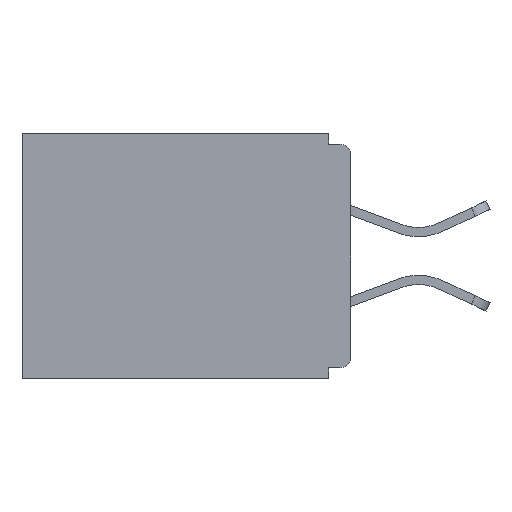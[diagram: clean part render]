
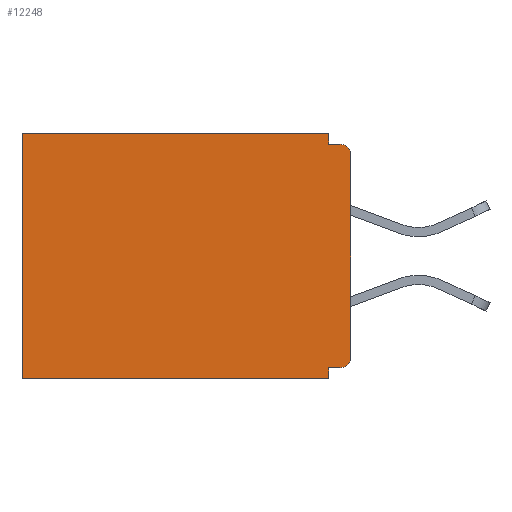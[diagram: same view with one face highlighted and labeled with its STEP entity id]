
A CAD part, left-side view. The second image highlights one B-rep face of the part: STEP entity #12248.
In plain terms, the highlighted planar face has unit normal (-1, 0, 0).
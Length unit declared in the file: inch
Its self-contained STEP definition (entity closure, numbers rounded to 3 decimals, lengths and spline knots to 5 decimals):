
#83 = LINE ( 'NONE', #18893, #19758 ) ;
#243 = PLANE ( 'NONE',  #15388 ) ;
#535 = CARTESIAN_POINT ( 'NONE',  ( 0.298, 0., 0. ) ) ;
#762 = CIRCLE ( 'NONE', #18149, 0.015 ) ;
#827 = CARTESIAN_POINT ( 'NONE',  ( 0.298, 0., -0.343 ) ) ;
#1192 = EDGE_CURVE ( 'NONE', #4054, #17444, #12206, .T. ) ;
#1280 = DIRECTION ( 'NONE',  ( -1., 0., 0. ) ) ;
#1309 = LINE ( 'NONE', #11753, #3973 ) ;
#1454 = VECTOR ( 'NONE', #13534, 39.37008 ) ;
#2074 = EDGE_CURVE ( 'NONE', #17963, #5428, #17317, .T. ) ;
#2093 = VERTEX_POINT ( 'NONE', #12678 ) ;
#2185 = DIRECTION ( 'NONE',  ( 0., 1., 0. ) ) ;
#2218 = DIRECTION ( 'NONE',  ( 1., 0., 0. ) ) ;
#2551 = EDGE_CURVE ( 'NONE', #17830, #2976, #13533, .T. ) ;
#2976 = VERTEX_POINT ( 'NONE', #8248 ) ;
#3218 = CARTESIAN_POINT ( 'NONE',  ( 0.298, 0.031, -0.343 ) ) ;
#3375 = EDGE_CURVE ( 'NONE', #14370, #2093, #15878, .T. ) ;
#3574 = VERTEX_POINT ( 'NONE', #3759 ) ;
#3759 = CARTESIAN_POINT ( 'NONE',  ( 0.298, 0., -0.313 ) ) ;
#3973 = VECTOR ( 'NONE', #4963, 39.37008 ) ;
#3991 = AXIS2_PLACEMENT_3D ( 'NONE', #20181, #1280, #9865 ) ;
#4046 = VECTOR ( 'NONE', #12881, 39.37008 ) ;
#4054 = VERTEX_POINT ( 'NONE', #20163 ) ;
#4190 = ORIENTED_EDGE ( 'NONE', *, *, #19865, .F. ) ;
#4683 = CARTESIAN_POINT ( 'NONE',  ( 0.298, 0.46, 0. ) ) ;
#4963 = DIRECTION ( 'NONE',  ( 0., 0., -1. ) ) ;
#5018 = ORIENTED_EDGE ( 'NONE', *, *, #2551, .F. ) ;
#5232 = EDGE_CURVE ( 'NONE', #16678, #17444, #12615, .T. ) ;
#5428 = VERTEX_POINT ( 'NONE', #4683 ) ;
#5670 = DIRECTION ( 'NONE',  ( 0., 0., -1. ) ) ;
#6103 = DIRECTION ( 'NONE',  ( 0., -1., 0. ) ) ;
#6512 = FACE_OUTER_BOUND ( 'NONE', #19383, .T. ) ;
#6931 = ORIENTED_EDGE ( 'NONE', *, *, #7677, .T. ) ;
#7677 = EDGE_CURVE ( 'NONE', #5428, #2976, #18415, .T. ) ;
#8248 = CARTESIAN_POINT ( 'NONE',  ( 0.298, 0.46, -0.343 ) ) ;
#8335 = CARTESIAN_POINT ( 'NONE',  ( 0.298, 0., 0. ) ) ;
#9244 = ORIENTED_EDGE ( 'NONE', *, *, #5232, .F. ) ;
#9865 = DIRECTION ( 'NONE',  ( 0., 0., -1. ) ) ;
#10078 = LINE ( 'NONE', #8335, #1454 ) ;
#10292 = ORIENTED_EDGE ( 'NONE', *, *, #2074, .T. ) ;
#11278 = CARTESIAN_POINT ( 'NONE',  ( 0.298, 0.46, 0. ) ) ;
#11389 = VECTOR ( 'NONE', #2185, 39.37008 ) ;
#11753 = CARTESIAN_POINT ( 'NONE',  ( 0.298, 0.031, -0.343 ) ) ;
#11965 = DIRECTION ( 'NONE',  ( 0., 0., -1. ) ) ;
#12206 = CIRCLE ( 'NONE', #3991, 0.015 ) ;
#12248 = ADVANCED_FACE ( 'NONE', ( #6512 ), #243, .F. ) ;
#12615 = LINE ( 'NONE', #14713, #21194 ) ;
#12678 = CARTESIAN_POINT ( 'NONE',  ( 0.298, 0.031, -0.328 ) ) ;
#12693 = VECTOR ( 'NONE', #16017, 39.37008 ) ;
#12827 = ORIENTED_EDGE ( 'NONE', *, *, #3375, .F. ) ;
#12881 = DIRECTION ( 'NONE',  ( 0., 1., 0. ) ) ;
#13533 = LINE ( 'NONE', #827, #4046 ) ;
#13534 = DIRECTION ( 'NONE',  ( 0., 0., -1. ) ) ;
#13902 = CARTESIAN_POINT ( 'NONE',  ( 0.298, 0.015, -0.313 ) ) ;
#13968 = DIRECTION ( 'NONE',  ( 0., 0., -1. ) ) ;
#14249 = ORIENTED_EDGE ( 'NONE', *, *, #14692, .F. ) ;
#14370 = VERTEX_POINT ( 'NONE', #19082 ) ;
#14379 = EDGE_CURVE ( 'NONE', #14370, #3574, #762, .T. ) ;
#14692 = EDGE_CURVE ( 'NONE', #2093, #17830, #1309, .T. ) ;
#14713 = CARTESIAN_POINT ( 'NONE',  ( 0.298, 0., -0.015 ) ) ;
#15388 = AXIS2_PLACEMENT_3D ( 'NONE', #535, #2218, #5670 ) ;
#15878 = LINE ( 'NONE', #17752, #12693 ) ;
#15969 = ORIENTED_EDGE ( 'NONE', *, *, #1192, .T. ) ;
#16017 = DIRECTION ( 'NONE',  ( 0., 1., 0. ) ) ;
#16678 = VERTEX_POINT ( 'NONE', #17539 ) ;
#17317 = LINE ( 'NONE', #21061, #11389 ) ;
#17444 = VERTEX_POINT ( 'NONE', #20456 ) ;
#17539 = CARTESIAN_POINT ( 'NONE',  ( 0.298, 0.031, -0.015 ) ) ;
#17752 = CARTESIAN_POINT ( 'NONE',  ( 0.298, 0., -0.328 ) ) ;
#17830 = VERTEX_POINT ( 'NONE', #3218 ) ;
#17963 = VERTEX_POINT ( 'NONE', #20294 ) ;
#18149 = AXIS2_PLACEMENT_3D ( 'NONE', #13902, #19372, #13968 ) ;
#18280 = DIRECTION ( 'NONE',  ( 0., 0., -1. ) ) ;
#18415 = LINE ( 'NONE', #11278, #21914 ) ;
#18893 = CARTESIAN_POINT ( 'NONE',  ( 0.298, 0.031, -0.343 ) ) ;
#19082 = CARTESIAN_POINT ( 'NONE',  ( 0.298, 0.015, -0.328 ) ) ;
#19372 = DIRECTION ( 'NONE',  ( -1., 0., 0. ) ) ;
#19383 = EDGE_LOOP ( 'NONE', ( #15969, #9244, #22145, #10292, #6931, #5018, #14249, #12827, #22054, #4190 ) ) ;
#19758 = VECTOR ( 'NONE', #11965, 39.37008 ) ;
#19865 = EDGE_CURVE ( 'NONE', #4054, #3574, #10078, .T. ) ;
#20163 = CARTESIAN_POINT ( 'NONE',  ( 0.298, 0., -0.03 ) ) ;
#20181 = CARTESIAN_POINT ( 'NONE',  ( 0.298, 0.015, -0.03 ) ) ;
#20294 = CARTESIAN_POINT ( 'NONE',  ( 0.298, 0.031, 0. ) ) ;
#20456 = CARTESIAN_POINT ( 'NONE',  ( 0.298, 0.015, -0.015 ) ) ;
#21061 = CARTESIAN_POINT ( 'NONE',  ( 0.298, 0., 0. ) ) ;
#21194 = VECTOR ( 'NONE', #6103, 39.37008 ) ;
#21914 = VECTOR ( 'NONE', #18280, 39.37008 ) ;
#22054 = ORIENTED_EDGE ( 'NONE', *, *, #14379, .T. ) ;
#22145 = ORIENTED_EDGE ( 'NONE', *, *, #22163, .F. ) ;
#22163 = EDGE_CURVE ( 'NONE', #17963, #16678, #83, .T. ) ;
